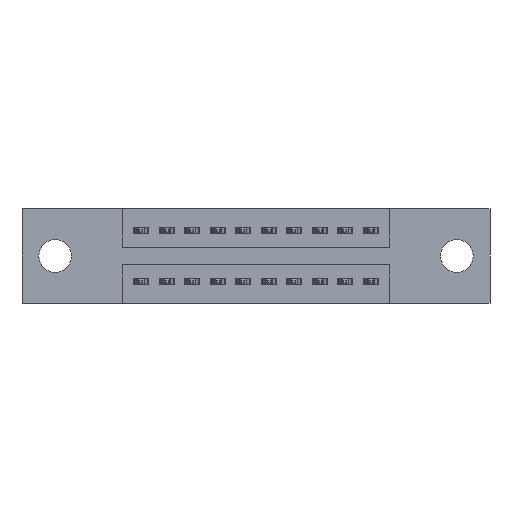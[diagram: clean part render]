
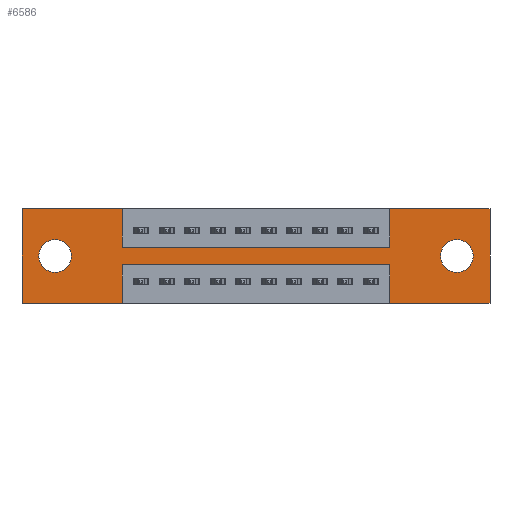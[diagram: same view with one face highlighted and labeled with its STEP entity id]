
A CAD part, front view. The second image highlights one B-rep face of the part: STEP entity #6586.
In plain terms, the highlighted planar face has unit normal (0, -1, 0).
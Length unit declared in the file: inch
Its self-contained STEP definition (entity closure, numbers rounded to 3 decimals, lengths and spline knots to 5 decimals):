
#64 = CARTESIAN_POINT ( 'NONE',  ( 1.4425, 0., -0.22 ) ) ;
#86 = CARTESIAN_POINT ( 'NONE',  ( 0., 0., 0. ) ) ;
#105 = FACE_BOUND ( 'NONE', #4207, .T. ) ;
#198 = AXIS2_PLACEMENT_3D ( 'NONE', #2864, #9456, #3845 ) ;
#276 = AXIS2_PLACEMENT_3D ( 'NONE', #2336, #5242, #11697 ) ;
#806 = ORIENTED_EDGE ( 'NONE', *, *, #12119, .F. ) ;
#838 = LINE ( 'NONE', #10479, #8168 ) ;
#973 = VECTOR ( 'NONE', #6870, 39.37008 ) ;
#1093 = VECTOR ( 'NONE', #5462, 39.37008 ) ;
#1164 = VECTOR ( 'NONE', #5808, 39.37008 ) ;
#1216 = VERTEX_POINT ( 'NONE', #9321 ) ;
#1256 = DIRECTION ( 'NONE',  ( 0., 0., -1. ) ) ;
#1283 = EDGE_CURVE ( 'NONE', #3211, #5938, #10899, .T. ) ;
#1511 = VECTOR ( 'NONE', #10500, 39.37008 ) ;
#1545 = CIRCLE ( 'NONE', #10766, 0.064 ) ;
#1550 = LINE ( 'NONE', #9413, #4439 ) ;
#1964 = CARTESIAN_POINT ( 'NONE',  ( 1.705, 0., -0.185 ) ) ;
#2046 = DIRECTION ( 'NONE',  ( 1., 0., 0. ) ) ;
#2047 = VECTOR ( 'NONE', #8159, 39.37008 ) ;
#2059 = CARTESIAN_POINT ( 'NONE',  ( 0., 0., 0. ) ) ;
#2277 = CARTESIAN_POINT ( 'NONE',  ( 0.3925, 0., 0. ) ) ;
#2336 = CARTESIAN_POINT ( 'NONE',  ( 0., 0., -0.37 ) ) ;
#2376 = EDGE_LOOP ( 'NONE', ( #4001, #806, #9872, #10157, #4313, #11989, #4006, #11434, #3421, #6221, #5057, #3100 ) ) ;
#2404 = FACE_OUTER_BOUND ( 'NONE', #2376, .T. ) ;
#2412 = EDGE_CURVE ( 'NONE', #4383, #2430, #11864, .T. ) ;
#2415 = CARTESIAN_POINT ( 'NONE',  ( 0.3925, 0., -0.22 ) ) ;
#2422 = VERTEX_POINT ( 'NONE', #7625 ) ;
#2430 = VERTEX_POINT ( 'NONE', #2458 ) ;
#2443 = VERTEX_POINT ( 'NONE', #64 ) ;
#2458 = CARTESIAN_POINT ( 'NONE',  ( 1.705, 0., -0.249 ) ) ;
#2566 = DIRECTION ( 'NONE',  ( 0., 0., 1. ) ) ;
#2574 = CARTESIAN_POINT ( 'NONE',  ( 1.835, 0., 0. ) ) ;
#2582 = VERTEX_POINT ( 'NONE', #9328 ) ;
#2658 = VECTOR ( 'NONE', #1256, 39.37008 ) ;
#2710 = CARTESIAN_POINT ( 'NONE',  ( 1.705, 0., -0.121 ) ) ;
#2759 = EDGE_LOOP ( 'NONE', ( #5642, #2778 ) ) ;
#2778 = ORIENTED_EDGE ( 'NONE', *, *, #10574, .T. ) ;
#2864 = CARTESIAN_POINT ( 'NONE',  ( 0.13, 0., -0.185 ) ) ;
#2889 = CARTESIAN_POINT ( 'NONE',  ( 0.13, 0., -0.185 ) ) ;
#2953 = DIRECTION ( 'NONE',  ( 0., 0., 1. ) ) ;
#2956 = DIRECTION ( 'NONE',  ( 0., 0., -1. ) ) ;
#3037 = VECTOR ( 'NONE', #10223, 39.37008 ) ;
#3100 = ORIENTED_EDGE ( 'NONE', *, *, #11871, .F. ) ;
#3158 = CARTESIAN_POINT ( 'NONE',  ( 0.3925, 0., -0.22 ) ) ;
#3211 = VERTEX_POINT ( 'NONE', #4630 ) ;
#3421 = ORIENTED_EDGE ( 'NONE', *, *, #8320, .F. ) ;
#3687 = CARTESIAN_POINT ( 'NONE',  ( 0., 0., -0.37 ) ) ;
#3845 = DIRECTION ( 'NONE',  ( 0., 0., 1. ) ) ;
#3858 = DIRECTION ( 'NONE',  ( 0., 0., 1. ) ) ;
#3873 = LINE ( 'NONE', #2059, #6077 ) ;
#3983 = LINE ( 'NONE', #2574, #1093 ) ;
#4001 = ORIENTED_EDGE ( 'NONE', *, *, #8207, .F. ) ;
#4006 = ORIENTED_EDGE ( 'NONE', *, *, #7650, .F. ) ;
#4033 = EDGE_CURVE ( 'NONE', #2422, #9329, #1550, .T. ) ;
#4207 = EDGE_LOOP ( 'NONE', ( #11846, #4620 ) ) ;
#4313 = ORIENTED_EDGE ( 'NONE', *, *, #10359, .F. ) ;
#4372 = AXIS2_PLACEMENT_3D ( 'NONE', #2889, #9471, #3858 ) ;
#4383 = VERTEX_POINT ( 'NONE', #2710 ) ;
#4439 = VECTOR ( 'NONE', #2566, 39.37008 ) ;
#4620 = ORIENTED_EDGE ( 'NONE', *, *, #9920, .T. ) ;
#4630 = CARTESIAN_POINT ( 'NONE',  ( 0.3925, 0., -0.15 ) ) ;
#4941 = DIRECTION ( 'NONE',  ( 1., 0., 0. ) ) ;
#4964 = FACE_BOUND ( 'NONE', #2759, .T. ) ;
#5057 = ORIENTED_EDGE ( 'NONE', *, *, #4033, .F. ) ;
#5197 = CARTESIAN_POINT ( 'NONE',  ( 1.835, 0., 0. ) ) ;
#5242 = DIRECTION ( 'NONE',  ( 0., -1., 0. ) ) ;
#5311 = DIRECTION ( 'NONE',  ( -1., 0., 0. ) ) ;
#5434 = VERTEX_POINT ( 'NONE', #8052 ) ;
#5462 = DIRECTION ( 'NONE',  ( 0., 0., -1. ) ) ;
#5517 = VERTEX_POINT ( 'NONE', #6238 ) ;
#5642 = ORIENTED_EDGE ( 'NONE', *, *, #2412, .T. ) ;
#5653 = EDGE_CURVE ( 'NONE', #5434, #7251, #7776, .T. ) ;
#5724 = CARTESIAN_POINT ( 'NONE',  ( 0.3925, 0., -0.15 ) ) ;
#5759 = CARTESIAN_POINT ( 'NONE',  ( 0., 0., 0. ) ) ;
#5808 = DIRECTION ( 'NONE',  ( 1., 0., 0. ) ) ;
#5900 = CARTESIAN_POINT ( 'NONE',  ( 0.3925, 0., -0.37 ) ) ;
#5938 = VERTEX_POINT ( 'NONE', #10765 ) ;
#6077 = VECTOR ( 'NONE', #4941, 39.37008 ) ;
#6221 = ORIENTED_EDGE ( 'NONE', *, *, #8201, .F. ) ;
#6238 = CARTESIAN_POINT ( 'NONE',  ( 1.4425, 0., 0. ) ) ;
#6586 = ADVANCED_FACE ( 'NONE', ( #4964, #105, #2404 ), #8974, .T. ) ;
#6604 = LINE ( 'NONE', #9583, #1511 ) ;
#6649 = VERTEX_POINT ( 'NONE', #10864 ) ;
#6870 = DIRECTION ( 'NONE',  ( 0., 0., -1. ) ) ;
#7251 = VERTEX_POINT ( 'NONE', #9081 ) ;
#7522 = EDGE_CURVE ( 'NONE', #2582, #1216, #11735, .T. ) ;
#7625 = CARTESIAN_POINT ( 'NONE',  ( 0., 0., -0.37 ) ) ;
#7650 = EDGE_CURVE ( 'NONE', #5938, #5517, #838, .T. ) ;
#7737 = VERTEX_POINT ( 'NONE', #3158 ) ;
#7776 = LINE ( 'NONE', #3687, #3037 ) ;
#7937 = EDGE_CURVE ( 'NONE', #7251, #2443, #9889, .T. ) ;
#8051 = DIRECTION ( 'NONE',  ( 0., 0., -1. ) ) ;
#8052 = CARTESIAN_POINT ( 'NONE',  ( 1.835, 0., -0.37 ) ) ;
#8105 = DIRECTION ( 'NONE',  ( 0., 1., 0. ) ) ;
#8159 = DIRECTION ( 'NONE',  ( 0., 0., 1. ) ) ;
#8168 = VECTOR ( 'NONE', #2953, 39.37008 ) ;
#8201 = EDGE_CURVE ( 'NONE', #9329, #6649, #3873, .T. ) ;
#8207 = EDGE_CURVE ( 'NONE', #7737, #9541, #11008, .T. ) ;
#8255 = LINE ( 'NONE', #86, #10678 ) ;
#8320 = EDGE_CURVE ( 'NONE', #6649, #3211, #9578, .T. ) ;
#8370 = VECTOR ( 'NONE', #5311, 39.37008 ) ;
#8636 = DIRECTION ( 'NONE',  ( 0., 1., 0. ) ) ;
#8974 = PLANE ( 'NONE',  #276 ) ;
#9081 = CARTESIAN_POINT ( 'NONE',  ( 1.4425, 0., -0.37 ) ) ;
#9321 = CARTESIAN_POINT ( 'NONE',  ( 0.13, 0., -0.249 ) ) ;
#9328 = CARTESIAN_POINT ( 'NONE',  ( 0.13, 0., -0.121 ) ) ;
#9329 = VERTEX_POINT ( 'NONE', #5759 ) ;
#9413 = CARTESIAN_POINT ( 'NONE',  ( 0., 0., 0. ) ) ;
#9456 = DIRECTION ( 'NONE',  ( 0., 1., 0. ) ) ;
#9471 = DIRECTION ( 'NONE',  ( 0., 1., 0. ) ) ;
#9541 = VERTEX_POINT ( 'NONE', #9884 ) ;
#9578 = LINE ( 'NONE', #2277, #2658 ) ;
#9583 = CARTESIAN_POINT ( 'NONE',  ( 0., 0., -0.37 ) ) ;
#9608 = AXIS2_PLACEMENT_3D ( 'NONE', #11206, #8105, #8051 ) ;
#9872 = ORIENTED_EDGE ( 'NONE', *, *, #7937, .F. ) ;
#9884 = CARTESIAN_POINT ( 'NONE',  ( 0.3925, 0., -0.37 ) ) ;
#9889 = LINE ( 'NONE', #10011, #2047 ) ;
#9920 = EDGE_CURVE ( 'NONE', #1216, #2582, #10674, .T. ) ;
#10011 = CARTESIAN_POINT ( 'NONE',  ( 1.4425, 0., -0.37 ) ) ;
#10157 = ORIENTED_EDGE ( 'NONE', *, *, #5653, .F. ) ;
#10223 = DIRECTION ( 'NONE',  ( -1., 0., 0. ) ) ;
#10359 = EDGE_CURVE ( 'NONE', #12078, #5434, #3983, .T. ) ;
#10479 = CARTESIAN_POINT ( 'NONE',  ( 1.4425, 0., 0. ) ) ;
#10500 = DIRECTION ( 'NONE',  ( -1., 0., 0. ) ) ;
#10574 = EDGE_CURVE ( 'NONE', #2430, #4383, #1545, .T. ) ;
#10633 = EDGE_CURVE ( 'NONE', #5517, #12078, #8255, .T. ) ;
#10674 = CIRCLE ( 'NONE', #4372, 0.064 ) ;
#10678 = VECTOR ( 'NONE', #2046, 39.37008 ) ;
#10765 = CARTESIAN_POINT ( 'NONE',  ( 1.4425, 0., -0.15 ) ) ;
#10766 = AXIS2_PLACEMENT_3D ( 'NONE', #1964, #8636, #2956 ) ;
#10791 = LINE ( 'NONE', #2415, #8370 ) ;
#10864 = CARTESIAN_POINT ( 'NONE',  ( 0.3925, 0., 0. ) ) ;
#10899 = LINE ( 'NONE', #5724, #1164 ) ;
#11008 = LINE ( 'NONE', #5900, #973 ) ;
#11206 = CARTESIAN_POINT ( 'NONE',  ( 1.705, 0., -0.185 ) ) ;
#11434 = ORIENTED_EDGE ( 'NONE', *, *, #1283, .F. ) ;
#11697 = DIRECTION ( 'NONE',  ( 0., 0., -1. ) ) ;
#11735 = CIRCLE ( 'NONE', #198, 0.064 ) ;
#11846 = ORIENTED_EDGE ( 'NONE', *, *, #7522, .T. ) ;
#11864 = CIRCLE ( 'NONE', #9608, 0.064 ) ;
#11871 = EDGE_CURVE ( 'NONE', #9541, #2422, #6604, .T. ) ;
#11989 = ORIENTED_EDGE ( 'NONE', *, *, #10633, .F. ) ;
#12078 = VERTEX_POINT ( 'NONE', #5197 ) ;
#12119 = EDGE_CURVE ( 'NONE', #2443, #7737, #10791, .T. ) ;
